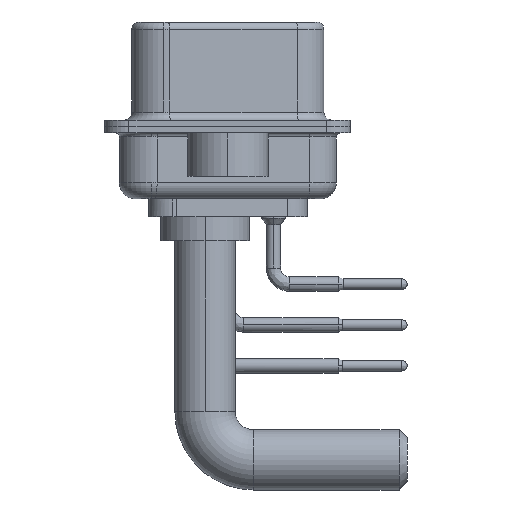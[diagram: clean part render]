
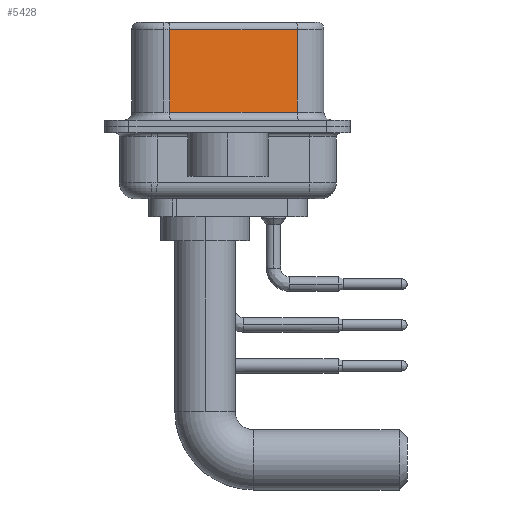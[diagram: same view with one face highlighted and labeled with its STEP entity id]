
A CAD part, left-side view. The second image highlights one B-rep face of the part: STEP entity #5428.
In plain terms, the highlighted planar face has unit normal (-0.985, -0.174, 0).
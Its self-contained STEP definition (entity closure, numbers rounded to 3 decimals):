
#1964 = CARTESIAN_POINT ( 'NONE',  ( 5.132, -4.322, 6.52 ) ) ;
#2707 = AXIS2_PLACEMENT_3D ( 'NONE', #1964, #23473, #31434 ) ;
#4300 = CARTESIAN_POINT ( 'NONE',  ( 5.132, -4.322, 6.02 ) ) ;
#4747 = FACE_OUTER_BOUND ( 'NONE', #17065, .T. ) ;
#5428 = ADVANCED_FACE ( 'NONE', ( #4747 ), #26233, .F. ) ;
#5758 = CARTESIAN_POINT ( 'NONE',  ( 5.132, -4.322, 6.52 ) ) ;
#6189 = DIRECTION ( 'NONE',  ( 0., 0., -1. ) ) ;
#6550 = LINE ( 'NONE', #4300, #16030 ) ;
#7035 = CARTESIAN_POINT ( 'NONE',  ( 5.132, -4.322, 0.9 ) ) ;
#7781 = CARTESIAN_POINT ( 'NONE',  ( 5.132, -4.322, 6.02 ) ) ;
#7782 = VERTEX_POINT ( 'NONE', #7781 ) ;
#10270 = VECTOR ( 'NONE', #13038, 1000. ) ;
#11118 = DIRECTION ( 'NONE',  ( 0., 0., -1. ) ) ;
#11389 = CARTESIAN_POINT ( 'NONE',  ( 3.73, 3.628, 6.52 ) ) ;
#13038 = DIRECTION ( 'NONE',  ( 0.174, -0.985, 0. ) ) ;
#13865 = EDGE_CURVE ( 'NONE', #7782, #32415, #22676, .T. ) ;
#13968 = LINE ( 'NONE', #11389, #33569 ) ;
#16030 = VECTOR ( 'NONE', #22321, 1000. ) ;
#16143 = LINE ( 'NONE', #26732, #10270 ) ;
#17065 = EDGE_LOOP ( 'NONE', ( #31119, #30194, #28897, #33291 ) ) ;
#17521 = VERTEX_POINT ( 'NONE', #33545 ) ;
#18044 = EDGE_CURVE ( 'NONE', #17521, #32415, #16143, .T. ) ;
#18999 = EDGE_CURVE ( 'NONE', #21031, #17521, #13968, .T. ) ;
#21031 = VERTEX_POINT ( 'NONE', #23354 ) ;
#22321 = DIRECTION ( 'NONE',  ( -0.174, 0.985, 0. ) ) ;
#22676 = LINE ( 'NONE', #5758, #27352 ) ;
#23354 = CARTESIAN_POINT ( 'NONE',  ( 3.73, 3.628, 6.02 ) ) ;
#23473 = DIRECTION ( 'NONE',  ( 0.985, 0.174, 0. ) ) ;
#23753 = EDGE_CURVE ( 'NONE', #7782, #21031, #6550, .T. ) ;
#26233 = PLANE ( 'NONE',  #2707 ) ;
#26732 = CARTESIAN_POINT ( 'NONE',  ( 5.132, -4.322, 0.9 ) ) ;
#27352 = VECTOR ( 'NONE', #11118, 1000. ) ;
#28897 = ORIENTED_EDGE ( 'NONE', *, *, #18999, .T. ) ;
#30194 = ORIENTED_EDGE ( 'NONE', *, *, #23753, .T. ) ;
#31119 = ORIENTED_EDGE ( 'NONE', *, *, #13865, .F. ) ;
#31434 = DIRECTION ( 'NONE',  ( -0.174, 0.985, 0. ) ) ;
#32415 = VERTEX_POINT ( 'NONE', #7035 ) ;
#33291 = ORIENTED_EDGE ( 'NONE', *, *, #18044, .T. ) ;
#33545 = CARTESIAN_POINT ( 'NONE',  ( 3.73, 3.628, 0.9 ) ) ;
#33569 = VECTOR ( 'NONE', #6189, 1000. ) ;
